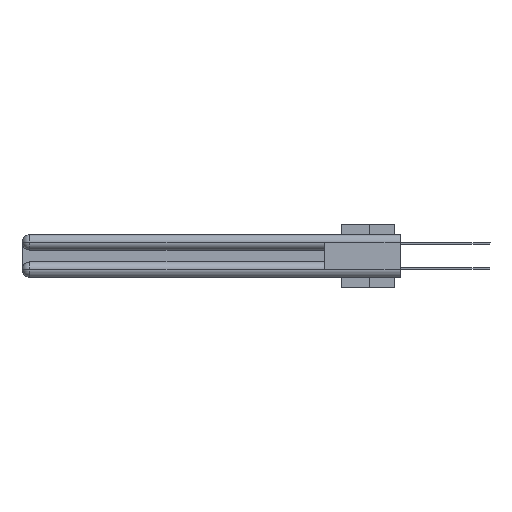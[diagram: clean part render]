
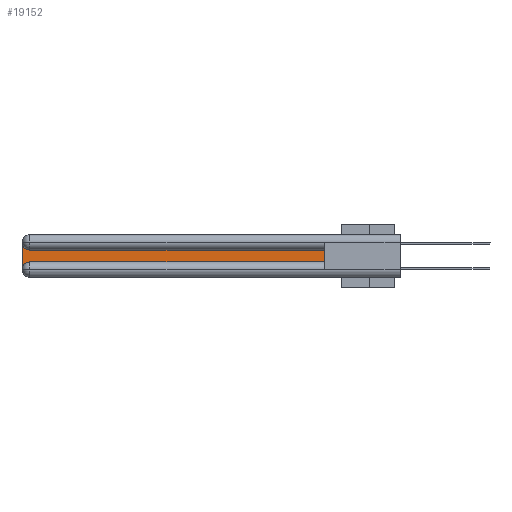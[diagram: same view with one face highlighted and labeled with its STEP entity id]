
A CAD part, left-side view. The second image highlights one B-rep face of the part: STEP entity #19152.
In plain terms, the highlighted planar face has unit normal (-1, 0, 0).
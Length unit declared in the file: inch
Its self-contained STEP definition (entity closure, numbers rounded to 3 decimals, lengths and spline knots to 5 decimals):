
#1340 = EDGE_CURVE ( 'NONE', #27813, #15638, #6611, .T. ) ;
#1911 = VERTEX_POINT ( 'NONE', #4323 ) ;
#1920 = VERTEX_POINT ( 'NONE', #34882 ) ;
#2572 = EDGE_CURVE ( 'NONE', #11032, #17218, #5016, .T. ) ;
#2664 = AXIS2_PLACEMENT_3D ( 'NONE', #9612, #15256, #4072 ) ;
#2706 = DIRECTION ( 'NONE',  ( 1., 0., 0. ) ) ;
#3825 = DIRECTION ( 'NONE',  ( 1., 0., 0. ) ) ;
#4072 = DIRECTION ( 'NONE',  ( 0., 0., -1. ) ) ;
#4323 = CARTESIAN_POINT ( 'NONE',  ( 0.075, 2.94, -0.2175 ) ) ;
#5016 = LINE ( 'NONE', #22033, #11847 ) ;
#5039 = LINE ( 'NONE', #16384, #32786 ) ;
#6611 = CIRCLE ( 'NONE', #35200, 0.06 ) ;
#6982 = CARTESIAN_POINT ( 'NONE',  ( 0.075, 0.6, -0.1225 ) ) ;
#7017 = CARTESIAN_POINT ( 'NONE',  ( 0.075, 2.94, -0.1225 ) ) ;
#7422 = LINE ( 'NONE', #26602, #8618 ) ;
#7956 = DIRECTION ( 'NONE',  ( 0., 0., 1. ) ) ;
#8618 = VECTOR ( 'NONE', #31911, 39.37008 ) ;
#9612 = CARTESIAN_POINT ( 'NONE',  ( 0.075, 2.94, -0.2775 ) ) ;
#9986 = ORIENTED_EDGE ( 'NONE', *, *, #17721, .T. ) ;
#11032 = VERTEX_POINT ( 'NONE', #33003 ) ;
#11847 = VECTOR ( 'NONE', #7956, 39.37008 ) ;
#12459 = DIRECTION ( 'NONE',  ( 0., 0., -1. ) ) ;
#12460 = AXIS2_PLACEMENT_3D ( 'NONE', #30674, #2706, #25386 ) ;
#12669 = EDGE_LOOP ( 'NONE', ( #27281, #13443, #15239, #33849, #9986, #32578 ) ) ;
#13443 = ORIENTED_EDGE ( 'NONE', *, *, #1340, .T. ) ;
#14426 = EDGE_CURVE ( 'NONE', #17218, #27813, #29820, .T. ) ;
#15239 = ORIENTED_EDGE ( 'NONE', *, *, #27414, .T. ) ;
#15256 = DIRECTION ( 'NONE',  ( 1., 0., 0. ) ) ;
#15638 = VERTEX_POINT ( 'NONE', #32022 ) ;
#16214 = DIRECTION ( 'NONE',  ( 0., -1., 0. ) ) ;
#16384 = CARTESIAN_POINT ( 'NONE',  ( 0.075, 0.6, -0.2175 ) ) ;
#17218 = VERTEX_POINT ( 'NONE', #6982 ) ;
#17721 = EDGE_CURVE ( 'NONE', #1911, #11032, #5039, .T. ) ;
#19152 = ADVANCED_FACE ( 'NONE', ( #19365 ), #33239, .F. ) ;
#19365 = FACE_OUTER_BOUND ( 'NONE', #12669, .T. ) ;
#20137 = CARTESIAN_POINT ( 'NONE',  ( 0.075, 2.94, -0.0625 ) ) ;
#22033 = CARTESIAN_POINT ( 'NONE',  ( 0.075, 0.6, -0.2175 ) ) ;
#23986 = DIRECTION ( 'NONE',  ( 0., 1., 0. ) ) ;
#25239 = EDGE_CURVE ( 'NONE', #1920, #1911, #26589, .T. ) ;
#25386 = DIRECTION ( 'NONE',  ( 0., 0., -1. ) ) ;
#26589 = CIRCLE ( 'NONE', #2664, 0.06 ) ;
#26602 = CARTESIAN_POINT ( 'NONE',  ( 0.075, 3., -0.2175 ) ) ;
#26718 = CARTESIAN_POINT ( 'NONE',  ( 0.075, 0.6, -0.1225 ) ) ;
#27281 = ORIENTED_EDGE ( 'NONE', *, *, #14426, .T. ) ;
#27414 = EDGE_CURVE ( 'NONE', #15638, #1920, #7422, .T. ) ;
#27813 = VERTEX_POINT ( 'NONE', #7017 ) ;
#29820 = LINE ( 'NONE', #26718, #30339 ) ;
#30339 = VECTOR ( 'NONE', #23986, 39.37008 ) ;
#30674 = CARTESIAN_POINT ( 'NONE',  ( 0.075, 3., -0.1225 ) ) ;
#31911 = DIRECTION ( 'NONE',  ( 0., 0., -1. ) ) ;
#32022 = CARTESIAN_POINT ( 'NONE',  ( 0.075, 3., -0.0625 ) ) ;
#32578 = ORIENTED_EDGE ( 'NONE', *, *, #2572, .T. ) ;
#32786 = VECTOR ( 'NONE', #16214, 39.37008 ) ;
#33003 = CARTESIAN_POINT ( 'NONE',  ( 0.075, 0.6, -0.2175 ) ) ;
#33239 = PLANE ( 'NONE',  #12460 ) ;
#33849 = ORIENTED_EDGE ( 'NONE', *, *, #25239, .T. ) ;
#34882 = CARTESIAN_POINT ( 'NONE',  ( 0.075, 3., -0.2775 ) ) ;
#35200 = AXIS2_PLACEMENT_3D ( 'NONE', #20137, #3825, #12459 ) ;
